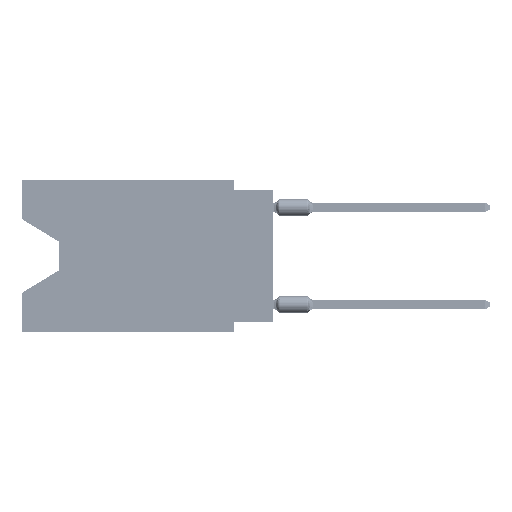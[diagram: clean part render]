
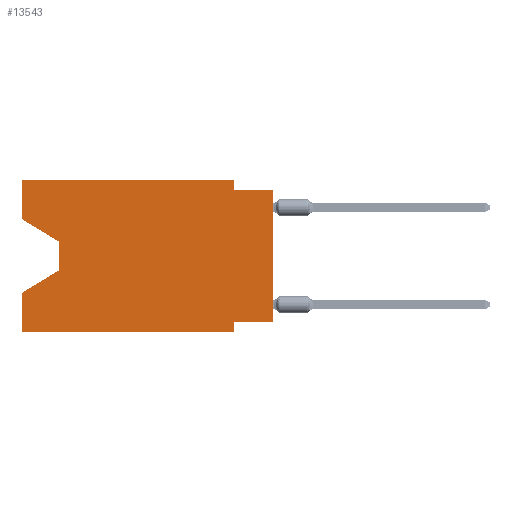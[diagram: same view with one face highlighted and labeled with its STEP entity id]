
A CAD part, left-side view. The second image highlights one B-rep face of the part: STEP entity #13543.
In plain terms, the highlighted planar face has unit normal (-1, 0, 0).
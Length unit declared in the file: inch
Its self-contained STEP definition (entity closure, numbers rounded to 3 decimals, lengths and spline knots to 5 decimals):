
#139 = LINE ( 'NONE', #45331, #49529 ) ;
#540 = ORIENTED_EDGE ( 'NONE', *, *, #52594, .F. ) ;
#1085 = DIRECTION ( 'NONE',  ( 0., 0.855, -0.519 ) ) ;
#1403 = CARTESIAN_POINT ( 'NONE',  ( 0., 0.1, 0. ) ) ;
#1451 = CARTESIAN_POINT ( 'NONE',  ( 0., 0.645, -0.39 ) ) ;
#1712 = VERTEX_POINT ( 'NONE', #64187 ) ;
#3377 = VERTEX_POINT ( 'NONE', #58944 ) ;
#4288 = DIRECTION ( 'NONE',  ( 0., 0., 1. ) ) ;
#4772 = ORIENTED_EDGE ( 'NONE', *, *, #12402, .T. ) ;
#6494 = CARTESIAN_POINT ( 'NONE',  ( 0., 0., -0.365 ) ) ;
#7185 = CARTESIAN_POINT ( 'NONE',  ( 0., 0.645, 0. ) ) ;
#9331 = CARTESIAN_POINT ( 'NONE',  ( 0., 0.55, -0.232 ) ) ;
#10026 = DIRECTION ( 'NONE',  ( 0., 0., 1. ) ) ;
#10198 = LINE ( 'NONE', #24097, #82607 ) ;
#10736 = VERTEX_POINT ( 'NONE', #9331 ) ;
#10806 = LINE ( 'NONE', #37293, #44891 ) ;
#12402 = EDGE_CURVE ( 'NONE', #10736, #49542, #53635, .T. ) ;
#12441 = FACE_OUTER_BOUND ( 'NONE', #80811, .T. ) ;
#13543 = ADVANCED_FACE ( 'NONE', ( #12441 ), #66691, .F. ) ;
#13583 = VERTEX_POINT ( 'NONE', #48002 ) ;
#14538 = CARTESIAN_POINT ( 'NONE',  ( 0., 0.55, -0.232 ) ) ;
#14712 = DIRECTION ( 'NONE',  ( 0., -1., 0. ) ) ;
#15108 = ORIENTED_EDGE ( 'NONE', *, *, #64720, .F. ) ;
#15640 = DIRECTION ( 'NONE',  ( 0., 0., -1. ) ) ;
#16859 = DIRECTION ( 'NONE',  ( 0., 0., 1. ) ) ;
#18257 = VECTOR ( 'NONE', #14712, 39.37008 ) ;
#19485 = ORIENTED_EDGE ( 'NONE', *, *, #42413, .T. ) ;
#19487 = ORIENTED_EDGE ( 'NONE', *, *, #72962, .T. ) ;
#20517 = DIRECTION ( 'NONE',  ( 0., 0., -1. ) ) ;
#22336 = CARTESIAN_POINT ( 'NONE',  ( 0., 0.645, -0.10025 ) ) ;
#22565 = VERTEX_POINT ( 'NONE', #6494 ) ;
#24029 = CARTESIAN_POINT ( 'NONE',  ( 0., 0.1, -0.365 ) ) ;
#24097 = CARTESIAN_POINT ( 'NONE',  ( 0., 0.645, -0.39 ) ) ;
#27228 = VECTOR ( 'NONE', #20517, 39.37008 ) ;
#28030 = DIRECTION ( 'NONE',  ( 0., 1., 0. ) ) ;
#28639 = CARTESIAN_POINT ( 'NONE',  ( 0., 0., -0.025 ) ) ;
#29589 = CARTESIAN_POINT ( 'NONE',  ( 0., 0.645, 0. ) ) ;
#30815 = VECTOR ( 'NONE', #16859, 39.37008 ) ;
#32069 = EDGE_CURVE ( 'NONE', #3377, #13583, #68170, .T. ) ;
#33678 = DIRECTION ( 'NONE',  ( 1., 0., 0. ) ) ;
#37293 = CARTESIAN_POINT ( 'NONE',  ( 0., 0., 0. ) ) ;
#37959 = DIRECTION ( 'NONE',  ( 0., -1., 0. ) ) ;
#38016 = ORIENTED_EDGE ( 'NONE', *, *, #81700, .F. ) ;
#38761 = CARTESIAN_POINT ( 'NONE',  ( 0., 0.645, -0.10025 ) ) ;
#39749 = CARTESIAN_POINT ( 'NONE',  ( 0., 0., -0.365 ) ) ;
#40908 = LINE ( 'NONE', #1403, #27228 ) ;
#41587 = CARTESIAN_POINT ( 'NONE',  ( 0., 0.645, 0. ) ) ;
#41760 = CARTESIAN_POINT ( 'NONE',  ( 0., 0.1, 0. ) ) ;
#42300 = DIRECTION ( 'NONE',  ( 0., -0.855, -0.519 ) ) ;
#42413 = EDGE_CURVE ( 'NONE', #22565, #13583, #10806, .T. ) ;
#42833 = ORIENTED_EDGE ( 'NONE', *, *, #78048, .T. ) ;
#44670 = VECTOR ( 'NONE', #53883, 39.37008 ) ;
#44891 = VECTOR ( 'NONE', #4288, 39.37008 ) ;
#45331 = CARTESIAN_POINT ( 'NONE',  ( 0., 0.645, 0. ) ) ;
#46271 = LINE ( 'NONE', #39749, #49416 ) ;
#47183 = VERTEX_POINT ( 'NONE', #38761 ) ;
#47799 = LINE ( 'NONE', #61709, #44670 ) ;
#48002 = CARTESIAN_POINT ( 'NONE',  ( 0., 0., -0.025 ) ) ;
#48241 = LINE ( 'NONE', #75191, #74032 ) ;
#49356 = CARTESIAN_POINT ( 'NONE',  ( 0., 0.645, -0.28975 ) ) ;
#49416 = VECTOR ( 'NONE', #28030, 39.37008 ) ;
#49529 = VECTOR ( 'NONE', #53537, 39.37008 ) ;
#49542 = VERTEX_POINT ( 'NONE', #49356 ) ;
#50288 = VERTEX_POINT ( 'NONE', #41760 ) ;
#52594 = EDGE_CURVE ( 'NONE', #50288, #3377, #40908, .T. ) ;
#53537 = DIRECTION ( 'NONE',  ( 0., -1., 0. ) ) ;
#53635 = LINE ( 'NONE', #14538, #56641 ) ;
#53883 = DIRECTION ( 'NONE',  ( 0., 0., -1. ) ) ;
#54004 = EDGE_CURVE ( 'NONE', #58479, #49542, #63006, .T. ) ;
#55987 = CARTESIAN_POINT ( 'NONE',  ( 0., 0.645, 0. ) ) ;
#56462 = VECTOR ( 'NONE', #10026, 39.37008 ) ;
#56641 = VECTOR ( 'NONE', #1085, 39.37008 ) ;
#58479 = VERTEX_POINT ( 'NONE', #1451 ) ;
#58700 = ORIENTED_EDGE ( 'NONE', *, *, #32069, .F. ) ;
#58944 = CARTESIAN_POINT ( 'NONE',  ( 0., 0.1, -0.025 ) ) ;
#60171 = DIRECTION ( 'NONE',  ( 0., 0., -1. ) ) ;
#60768 = AXIS2_PLACEMENT_3D ( 'NONE', #7185, #33678, #60171 ) ;
#61709 = CARTESIAN_POINT ( 'NONE',  ( 0., 0.55, -0.158 ) ) ;
#62306 = LINE ( 'NONE', #22336, #62844 ) ;
#62844 = VECTOR ( 'NONE', #42300, 39.37008 ) ;
#63006 = LINE ( 'NONE', #29589, #56462 ) ;
#63755 = CARTESIAN_POINT ( 'NONE',  ( 0., 0.1, -0.39 ) ) ;
#64187 = CARTESIAN_POINT ( 'NONE',  ( 0., 0.55, -0.158 ) ) ;
#64720 = EDGE_CURVE ( 'NONE', #47183, #81105, #68586, .T. ) ;
#66691 = PLANE ( 'NONE',  #60768 ) ;
#66987 = ORIENTED_EDGE ( 'NONE', *, *, #75877, .F. ) ;
#67113 = EDGE_CURVE ( 'NONE', #1712, #10736, #47799, .T. ) ;
#68170 = LINE ( 'NONE', #28639, #18257 ) ;
#68586 = LINE ( 'NONE', #55987, #30815 ) ;
#69638 = ORIENTED_EDGE ( 'NONE', *, *, #67113, .T. ) ;
#69857 = ORIENTED_EDGE ( 'NONE', *, *, #78940, .F. ) ;
#72962 = EDGE_CURVE ( 'NONE', #47183, #1712, #62306, .T. ) ;
#74032 = VECTOR ( 'NONE', #15640, 39.37008 ) ;
#75191 = CARTESIAN_POINT ( 'NONE',  ( 0., 0.1, -0.39 ) ) ;
#75877 = EDGE_CURVE ( 'NONE', #76797, #82436, #48241, .T. ) ;
#76797 = VERTEX_POINT ( 'NONE', #24029 ) ;
#78048 = EDGE_CURVE ( 'NONE', #58479, #82436, #10198, .T. ) ;
#78940 = EDGE_CURVE ( 'NONE', #22565, #76797, #46271, .T. ) ;
#80060 = ORIENTED_EDGE ( 'NONE', *, *, #54004, .F. ) ;
#80811 = EDGE_LOOP ( 'NONE', ( #19487, #69638, #4772, #80060, #42833, #66987, #69857, #19485, #58700, #540, #38016, #15108 ) ) ;
#81105 = VERTEX_POINT ( 'NONE', #41587 ) ;
#81700 = EDGE_CURVE ( 'NONE', #81105, #50288, #139, .T. ) ;
#82436 = VERTEX_POINT ( 'NONE', #63755 ) ;
#82607 = VECTOR ( 'NONE', #37959, 39.37008 ) ;
